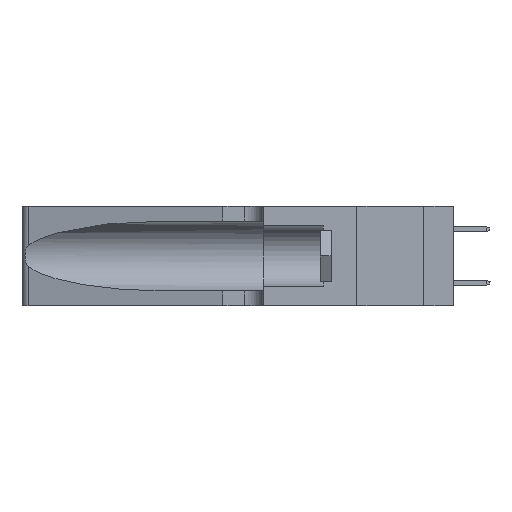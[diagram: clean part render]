
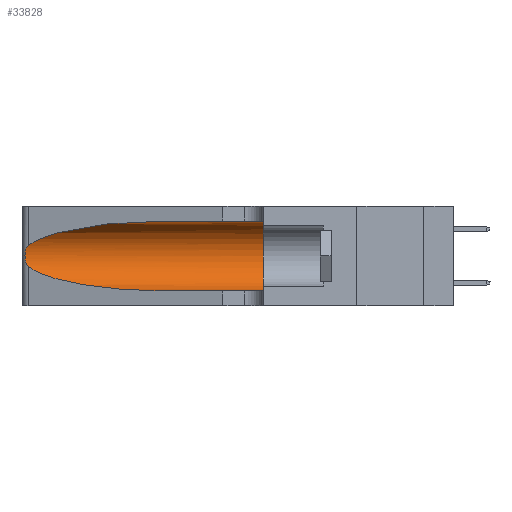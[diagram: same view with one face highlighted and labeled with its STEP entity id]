
A CAD part, left-side view. The second image highlights one B-rep face of the part: STEP entity #33828.
In plain terms, the highlighted cylindrical face has radius 3.308 mm (diameter 6.617 mm), a partial arc.
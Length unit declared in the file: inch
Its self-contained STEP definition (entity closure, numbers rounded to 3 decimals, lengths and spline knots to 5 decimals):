
#407 = EDGE_CURVE ( 'NONE', #37608, #23148, #11057, .T. ) ;
#1267 = CARTESIAN_POINT ( 'NONE',  ( 0.1305, 0.72297, 0.05475 ) ) ;
#2052 = VERTEX_POINT ( 'NONE', #26625 ) ;
#2500 = CARTESIAN_POINT ( 'NONE',  ( 0.26017, 1.23833, 0.17102 ) ) ;
#2686 =( BOUNDED_CURVE ( )  B_SPLINE_CURVE ( 3, ( #9965, #13407, #13826, #32910 ),
 .UNSPECIFIED., .F., .T. ) 
 B_SPLINE_CURVE_WITH_KNOTS ( ( 4, 4 ),
 ( 3.44316, 4.71239 ),
 .UNSPECIFIED. ) 
 CURVE ( )  GEOMETRIC_REPRESENTATION_ITEM ( )  RATIONAL_B_SPLINE_CURVE ( ( 1., 0.87, 0.87, 1. ) ) 
 REPRESENTATION_ITEM ( '' )  );
#3796 = CARTESIAN_POINT ( 'NONE',  ( 0.2373, 1.15595, 0.28018 ) ) ;
#4720 = VERTEX_POINT ( 'NONE', #13878 ) ;
#5139 = CARTESIAN_POINT ( 'NONE',  ( 0.25487, 1.22718, 0.22369 ) ) ;
#5940 = CARTESIAN_POINT ( 'NONE',  ( 0.25856, 1.23593, 0.16098 ) ) ;
#6363 = CARTESIAN_POINT ( 'NONE',  ( 0.25487, 1.22718, 0.14631 ) ) ;
#6559 = CARTESIAN_POINT ( 'NONE',  ( 0.1305, 1.61858, 0.31525 ) ) ;
#6567 = CARTESIAN_POINT ( 'NONE',  ( 0.1305, 0.35, 0.05475 ) ) ;
#6572 = CARTESIAN_POINT ( 'NONE',  ( 0.25555, 1.22994, 0.2215 ) ) ;
#6940 = EDGE_CURVE ( 'NONE', #33031, #23148, #28698, .T. ) ;
#7192 = DIRECTION ( 'NONE',  ( 0., 0., -1. ) ) ;
#8348 = EDGE_CURVE ( 'NONE', #22053, #37608, #35996, .T. ) ;
#9965 = CARTESIAN_POINT ( 'NONE',  ( 0.25487, 1.22718, 0.14631 ) ) ;
#11057 = CIRCLE ( 'NONE', #34338, 0.13025 ) ;
#11282 = CARTESIAN_POINT ( 'NONE',  ( 0.1305, 0.72297, 0.31525 ) ) ;
#11757 = DIRECTION ( 'NONE',  ( 0., -1., 0. ) ) ;
#12392 = CARTESIAN_POINT ( 'NONE',  ( 0.1305, 1.61858, 0.05475 ) ) ;
#12973 = VECTOR ( 'NONE', #11757, 39.37008 ) ;
#13407 = CARTESIAN_POINT ( 'NONE',  ( 0.2373, 1.15595, 0.08982 ) ) ;
#13457 = CARTESIAN_POINT ( 'NONE',  ( 0.1305, 1.61858, 0.185 ) ) ;
#13826 = CARTESIAN_POINT ( 'NONE',  ( 0.18966, 0.96281, 0.05475 ) ) ;
#13878 = CARTESIAN_POINT ( 'NONE',  ( 0.25487, 1.22718, 0.22369 ) ) ;
#15057 = CARTESIAN_POINT ( 'NONE',  ( 0.1305, 0.35, 0.31525 ) ) ;
#15213 = B_SPLINE_CURVE_WITH_KNOTS ( 'NONE', 3,
 ( #5139, #6572, #26136, #39053, #18263, #22691, #15829, #31341, #2500, #5940, #15616, #41861, #25502, #6363 ),
 .UNSPECIFIED., .F., .F.,
 ( 4, 2, 2, 2, 2, 2, 4 ),
 ( 0., 0.00027, 0.00053, 0.00107, 0.0016, 0.00187, 0.00214 ),
 .UNSPECIFIED. ) ;
#15381 = DIRECTION ( 'NONE',  ( 0., -1., 0. ) ) ;
#15616 = CARTESIAN_POINT ( 'NONE',  ( 0.25789, 1.23486, 0.15765 ) ) ;
#15755 = EDGE_LOOP ( 'NONE', ( #23585, #36904, #22289, #39893, #32736, #25797 ) ) ;
#15829 = CARTESIAN_POINT ( 'NONE',  ( 0.26075, 1.23896, 0.19203 ) ) ;
#16354 = CARTESIAN_POINT ( 'NONE',  ( 0.1305, 0.35, 0.185 ) ) ;
#16871 = DIRECTION ( 'NONE',  ( 0., -1., 0. ) ) ;
#18263 = CARTESIAN_POINT ( 'NONE',  ( 0.25854, 1.2359, 0.20912 ) ) ;
#22053 = VERTEX_POINT ( 'NONE', #11282 ) ;
#22135 = AXIS2_PLACEMENT_3D ( 'NONE', #13457, #16871, #7192 ) ;
#22289 = ORIENTED_EDGE ( 'NONE', *, *, #23838, .T. ) ;
#22691 = CARTESIAN_POINT ( 'NONE',  ( 0.26018, 1.23835, 0.19895 ) ) ;
#23148 = VERTEX_POINT ( 'NONE', #6567 ) ;
#23585 = ORIENTED_EDGE ( 'NONE', *, *, #26827, .T. ) ;
#23811 = CARTESIAN_POINT ( 'NONE',  ( 0.1305, 0.72297, 0.31525 ) ) ;
#23838 = EDGE_CURVE ( 'NONE', #2052, #33031, #2686, .T. ) ;
#24011 = CARTESIAN_POINT ( 'NONE',  ( 0.18966, 0.96281, 0.31525 ) ) ;
#25502 = CARTESIAN_POINT ( 'NONE',  ( 0.25555, 1.22993, 0.14849 ) ) ;
#25797 = ORIENTED_EDGE ( 'NONE', *, *, #8348, .F. ) ;
#26136 = CARTESIAN_POINT ( 'NONE',  ( 0.25639, 1.23184, 0.21858 ) ) ;
#26228 = DIRECTION ( 'NONE',  ( 0., 0., 1. ) ) ;
#26625 = CARTESIAN_POINT ( 'NONE',  ( 0.25487, 1.22718, 0.14631 ) ) ;
#26827 = EDGE_CURVE ( 'NONE', #22053, #4720, #34528, .T. ) ;
#28698 = LINE ( 'NONE', #12392, #12973 ) ;
#30179 = CYLINDRICAL_SURFACE ( 'NONE', #22135, 0.13025 ) ;
#31341 = CARTESIAN_POINT ( 'NONE',  ( 0.26075, 1.23896, 0.178 ) ) ;
#32736 = ORIENTED_EDGE ( 'NONE', *, *, #407, .F. ) ;
#32910 = CARTESIAN_POINT ( 'NONE',  ( 0.1305, 0.72297, 0.05475 ) ) ;
#33031 = VERTEX_POINT ( 'NONE', #1267 ) ;
#33828 = ADVANCED_FACE ( 'NONE', ( #36436 ), #30179, .F. ) ;
#34338 = AXIS2_PLACEMENT_3D ( 'NONE', #16354, #35681, #26228 ) ;
#34528 =( BOUNDED_CURVE ( )  B_SPLINE_CURVE ( 3, ( #23811, #24011, #3796, #40346 ),
 .UNSPECIFIED., .F., .T. ) 
 B_SPLINE_CURVE_WITH_KNOTS ( ( 4, 4 ),
 ( 1.5708, 2.84003 ),
 .UNSPECIFIED. ) 
 CURVE ( )  GEOMETRIC_REPRESENTATION_ITEM ( )  RATIONAL_B_SPLINE_CURVE ( ( 1., 0.87, 0.87, 1. ) ) 
 REPRESENTATION_ITEM ( '' )  );
#35681 = DIRECTION ( 'NONE',  ( 0., 1., 0. ) ) ;
#35996 = LINE ( 'NONE', #6559, #39813 ) ;
#36436 = FACE_OUTER_BOUND ( 'NONE', #15755, .T. ) ;
#36904 = ORIENTED_EDGE ( 'NONE', *, *, #39081, .T. ) ;
#37608 = VERTEX_POINT ( 'NONE', #15057 ) ;
#39053 = CARTESIAN_POINT ( 'NONE',  ( 0.25787, 1.23484, 0.2124 ) ) ;
#39081 = EDGE_CURVE ( 'NONE', #4720, #2052, #15213, .T. ) ;
#39813 = VECTOR ( 'NONE', #15381, 39.37008 ) ;
#39893 = ORIENTED_EDGE ( 'NONE', *, *, #6940, .T. ) ;
#40346 = CARTESIAN_POINT ( 'NONE',  ( 0.25487, 1.22718, 0.22369 ) ) ;
#41861 = CARTESIAN_POINT ( 'NONE',  ( 0.25639, 1.23186, 0.15144 ) ) ;
